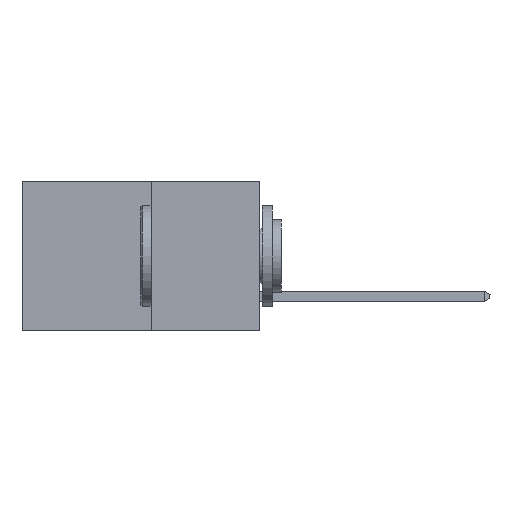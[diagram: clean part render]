
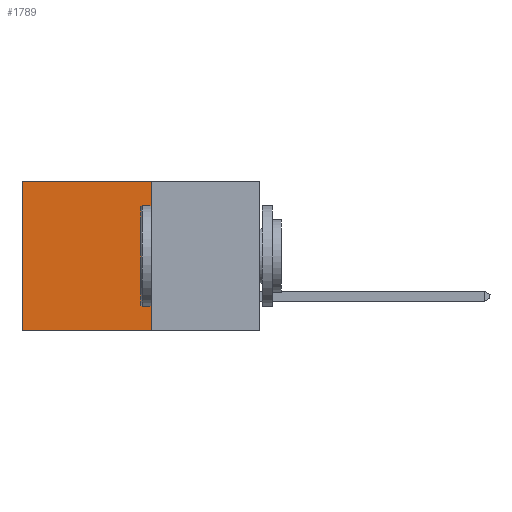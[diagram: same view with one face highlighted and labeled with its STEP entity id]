
A CAD part, left-side view. The second image highlights one B-rep face of the part: STEP entity #1789.
In plain terms, the highlighted planar face has unit normal (-1, 0, 0).
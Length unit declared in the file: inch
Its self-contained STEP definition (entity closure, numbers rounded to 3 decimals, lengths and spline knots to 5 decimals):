
#81 = DIRECTION ( 'NONE',  ( 0., 0., -1. ) ) ;
#755 = EDGE_CURVE ( 'NONE', #6739, #8986, #9911, .T. ) ;
#1171 = CARTESIAN_POINT ( 'NONE',  ( 0.277, 0.27, -0.37 ) ) ;
#1737 = VECTOR ( 'NONE', #9938, 39.37008 ) ;
#1789 = ADVANCED_FACE ( 'NONE', ( #1844 ), #8104, .F. ) ;
#1844 = FACE_OUTER_BOUND ( 'NONE', #5496, .T. ) ;
#2238 = CARTESIAN_POINT ( 'NONE',  ( 0.277, 0.27, 0. ) ) ;
#2638 = ORIENTED_EDGE ( 'NONE', *, *, #8356, .T. ) ;
#2708 = ORIENTED_EDGE ( 'NONE', *, *, #3725, .F. ) ;
#2721 = ORIENTED_EDGE ( 'NONE', *, *, #3844, .F. ) ;
#2741 = LINE ( 'NONE', #8931, #9550 ) ;
#2835 = DIRECTION ( 'NONE',  ( 1., 0., 0. ) ) ;
#2854 = ORIENTED_EDGE ( 'NONE', *, *, #755, .T. ) ;
#2966 = CARTESIAN_POINT ( 'NONE',  ( 0.277, 0.27, 0. ) ) ;
#3154 = VECTOR ( 'NONE', #3303, 39.37008 ) ;
#3303 = DIRECTION ( 'NONE',  ( 0., 1., 0. ) ) ;
#3503 = VECTOR ( 'NONE', #7571, 39.37008 ) ;
#3725 = EDGE_CURVE ( 'NONE', #6097, #7568, #6182, .T. ) ;
#3789 = LINE ( 'NONE', #7357, #3503 ) ;
#3844 = EDGE_CURVE ( 'NONE', #6739, #6097, #2741, .T. ) ;
#5359 = AXIS2_PLACEMENT_3D ( 'NONE', #5706, #2835, #81 ) ;
#5496 = EDGE_LOOP ( 'NONE', ( #2638, #2708, #2721, #2854 ) ) ;
#5706 = CARTESIAN_POINT ( 'NONE',  ( 0.277, 0.27, -0.37 ) ) ;
#5879 = CARTESIAN_POINT ( 'NONE',  ( 0.277, 0.59, 0. ) ) ;
#6097 = VERTEX_POINT ( 'NONE', #1171 ) ;
#6182 = LINE ( 'NONE', #9961, #1737 ) ;
#6739 = VERTEX_POINT ( 'NONE', #2966 ) ;
#7357 = CARTESIAN_POINT ( 'NONE',  ( 0.277, 0.59, -0.37 ) ) ;
#7568 = VERTEX_POINT ( 'NONE', #10942 ) ;
#7571 = DIRECTION ( 'NONE',  ( 0., 0., -1. ) ) ;
#8104 = PLANE ( 'NONE',  #5359 ) ;
#8356 = EDGE_CURVE ( 'NONE', #8986, #7568, #3789, .T. ) ;
#8891 = DIRECTION ( 'NONE',  ( 0., 0., -1. ) ) ;
#8931 = CARTESIAN_POINT ( 'NONE',  ( 0.277, 0.27, -0.37 ) ) ;
#8986 = VERTEX_POINT ( 'NONE', #5879 ) ;
#9550 = VECTOR ( 'NONE', #8891, 39.37008 ) ;
#9911 = LINE ( 'NONE', #2238, #3154 ) ;
#9938 = DIRECTION ( 'NONE',  ( 0., 1., 0. ) ) ;
#9961 = CARTESIAN_POINT ( 'NONE',  ( 0.277, 0.27, -0.37 ) ) ;
#10942 = CARTESIAN_POINT ( 'NONE',  ( 0.277, 0.59, -0.37 ) ) ;
